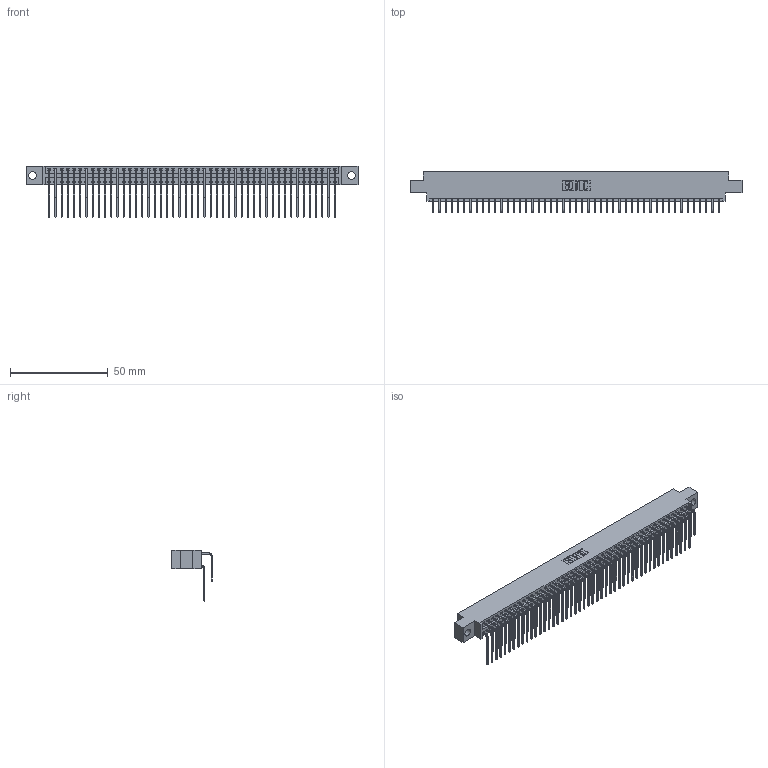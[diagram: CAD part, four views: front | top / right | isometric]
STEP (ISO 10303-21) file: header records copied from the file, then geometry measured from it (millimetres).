
FILE_DESCRIPTION (( 'STEP AP203' ), '1' );
FILE_NAME ('346-094-559-804.STEP', '2018-08-30T06:02:20', ( '' ), ( '' ), 'SwSTEP 2.0', 'SolidWorks 2016', '' );
FILE_SCHEMA (( 'CONFIG_CONTROL_DESIGN' ));
Length unit declared in the file: inch
Products named in the file (4): 346 Part_0.170 Offset - 0.156 Dia-TH; 345-292-001_558 559 Tail - 1; 345-292-001_559 Tail - 2; 346-094-559-804
Assembly tree (95 placements, depth 2):
  346-094-559-804
    346 Part_0.170 Offset - 0.156 Dia-TH
    345-292-001_558 559 Tail - 1  x47
    345-292-001_559 Tail - 2  x47
Bounding box: 169.8 x 20.89 x 26.16 mm (x, y, z)
Volume: 16896.1 mm3; surface area: 25897.9 mm2
Topology: 95 solids, 95 shells, 5202 faces, 15475 edges, 10190 vertices
Faces by surface type: plane 3558, cylinder 1644
Entity records: 31919 total; most frequent: CARTESIAN_POINT 5307, ORIENTED_EDGE 5190, DIRECTION 4699, EDGE_CURVE 2595, LINE 2235, VECTOR 2235, VERTEX_POINT 1726, AXIS2_PLACEMENT_3D 1232
